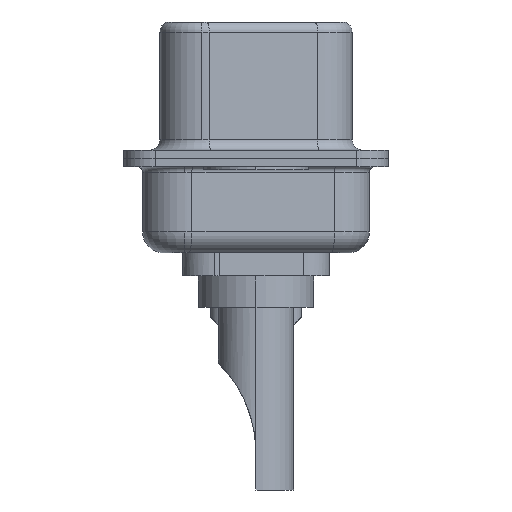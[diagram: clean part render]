
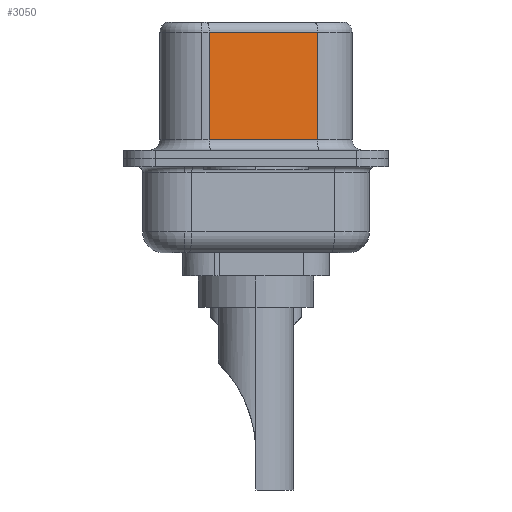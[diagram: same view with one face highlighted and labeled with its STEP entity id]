
A CAD part, left-side view. The second image highlights one B-rep face of the part: STEP entity #3050.
In plain terms, the highlighted planar face has unit normal (-0.985, -0.174, 0).
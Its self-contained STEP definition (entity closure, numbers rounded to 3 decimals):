
#97 = LINE ( 'NONE', #9679, #13910 ) ;
#456 = CARTESIAN_POINT ( 'NONE',  ( 4.585, -2.927, 6.52 ) ) ;
#844 = DIRECTION ( 'NONE',  ( 0., 0., -1. ) ) ;
#1031 = DIRECTION ( 'NONE',  ( -0.174, 0.985, 0. ) ) ;
#1068 = EDGE_CURVE ( 'NONE', #1667, #5191, #4103, .T. ) ;
#1667 = VERTEX_POINT ( 'NONE', #7553 ) ;
#3050 = ADVANCED_FACE ( 'NONE', ( #11850 ), #8675, .F. ) ;
#3163 = EDGE_CURVE ( 'NONE', #1667, #15460, #5994, .T. ) ;
#3607 = CARTESIAN_POINT ( 'NONE',  ( 4.585, -2.927, 0.9 ) ) ;
#3937 = AXIS2_PLACEMENT_3D ( 'NONE', #8558, #8692, #15312 ) ;
#4103 = LINE ( 'NONE', #456, #10641 ) ;
#5191 = VERTEX_POINT ( 'NONE', #3607 ) ;
#5827 = EDGE_CURVE ( 'NONE', #15460, #10439, #17811, .T. ) ;
#5994 = LINE ( 'NONE', #8118, #12947 ) ;
#7553 = CARTESIAN_POINT ( 'NONE',  ( 4.585, -2.927, 6.02 ) ) ;
#8118 = CARTESIAN_POINT ( 'NONE',  ( 4.585, -2.927, 6.02 ) ) ;
#8558 = CARTESIAN_POINT ( 'NONE',  ( 4.585, -2.927, 6.52 ) ) ;
#8675 = PLANE ( 'NONE',  #3937 ) ;
#8692 = DIRECTION ( 'NONE',  ( 0.985, 0.174, 0. ) ) ;
#9276 = ORIENTED_EDGE ( 'NONE', *, *, #1068, .F. ) ;
#9679 = CARTESIAN_POINT ( 'NONE',  ( 4.585, -2.927, 0.9 ) ) ;
#9779 = DIRECTION ( 'NONE',  ( 0., 0., -1. ) ) ;
#10439 = VERTEX_POINT ( 'NONE', #12588 ) ;
#10641 = VECTOR ( 'NONE', #9779, 1000. ) ;
#11850 = FACE_OUTER_BOUND ( 'NONE', #13321, .T. ) ;
#12452 = DIRECTION ( 'NONE',  ( 0.174, -0.985, 0. ) ) ;
#12588 = CARTESIAN_POINT ( 'NONE',  ( 3.675, 2.233, 0.9 ) ) ;
#12589 = ORIENTED_EDGE ( 'NONE', *, *, #3163, .T. ) ;
#12947 = VECTOR ( 'NONE', #1031, 1000. ) ;
#13230 = CARTESIAN_POINT ( 'NONE',  ( 3.675, 2.233, 6.52 ) ) ;
#13321 = EDGE_LOOP ( 'NONE', ( #9276, #12589, #16947, #15407 ) ) ;
#13910 = VECTOR ( 'NONE', #12452, 1000. ) ;
#14069 = VECTOR ( 'NONE', #844, 1000. ) ;
#14408 = EDGE_CURVE ( 'NONE', #10439, #5191, #97, .T. ) ;
#14898 = CARTESIAN_POINT ( 'NONE',  ( 3.675, 2.233, 6.02 ) ) ;
#15312 = DIRECTION ( 'NONE',  ( -0.174, 0.985, 0. ) ) ;
#15407 = ORIENTED_EDGE ( 'NONE', *, *, #14408, .T. ) ;
#15460 = VERTEX_POINT ( 'NONE', #14898 ) ;
#16947 = ORIENTED_EDGE ( 'NONE', *, *, #5827, .T. ) ;
#17811 = LINE ( 'NONE', #13230, #14069 ) ;
